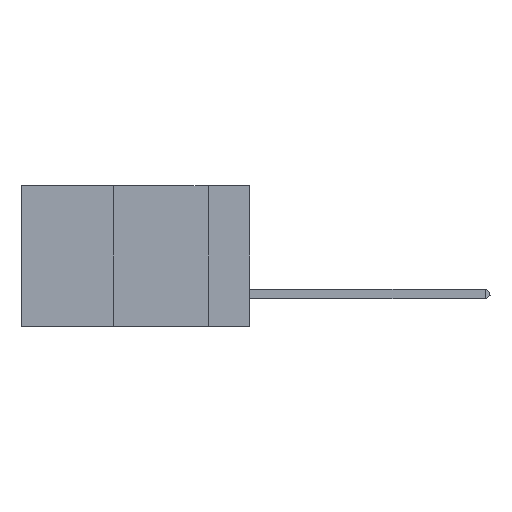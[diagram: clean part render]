
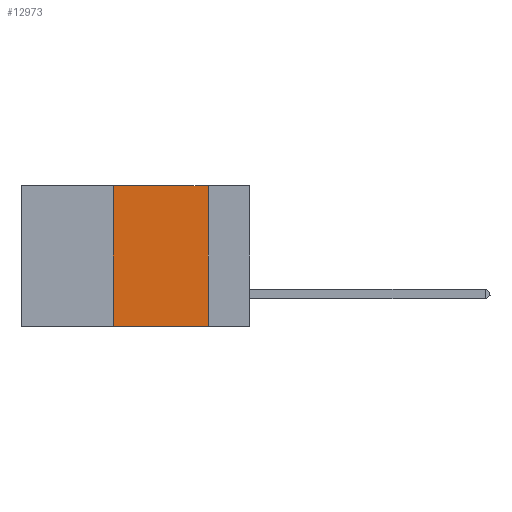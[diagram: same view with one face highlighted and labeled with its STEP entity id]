
A CAD part, left-side view. The second image highlights one B-rep face of the part: STEP entity #12973.
In plain terms, the highlighted planar face has unit normal (-1, 0, 0).
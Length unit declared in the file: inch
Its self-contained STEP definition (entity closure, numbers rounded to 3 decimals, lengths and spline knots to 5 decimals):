
#268 = ORIENTED_EDGE ( 'NONE', *, *, #5433, .F. ) ;
#937 = AXIS2_PLACEMENT_3D ( 'NONE', #36667, #13657, #36542 ) ;
#2885 = FACE_OUTER_BOUND ( 'NONE', #14887, .T. ) ;
#4518 = LINE ( 'NONE', #21459, #18249 ) ;
#5433 = EDGE_CURVE ( 'NONE', #33596, #33180, #33106, .T. ) ;
#8231 = DIRECTION ( 'NONE',  ( 0., 0., 1. ) ) ;
#8996 = CARTESIAN_POINT ( 'NONE',  ( 0., 0.6, -0.37 ) ) ;
#9204 = DIRECTION ( 'NONE',  ( 0., 0., -1. ) ) ;
#9628 = CARTESIAN_POINT ( 'NONE',  ( 0., 0.36, 0. ) ) ;
#11855 = VERTEX_POINT ( 'NONE', #20778 ) ;
#12973 = ADVANCED_FACE ( 'NONE', ( #2885 ), #30639, .F. ) ;
#13657 = DIRECTION ( 'NONE',  ( 1., 0., 0. ) ) ;
#14887 = EDGE_LOOP ( 'NONE', ( #19943, #26141, #268, #23049 ) ) ;
#16085 = VECTOR ( 'NONE', #9204, 39.37008 ) ;
#16979 = VERTEX_POINT ( 'NONE', #28825 ) ;
#18249 = VECTOR ( 'NONE', #24515, 39.37008 ) ;
#19943 = ORIENTED_EDGE ( 'NONE', *, *, #33631, .F. ) ;
#20144 = VECTOR ( 'NONE', #29435, 39.37008 ) ;
#20778 = CARTESIAN_POINT ( 'NONE',  ( 0., 0.11, -0.37 ) ) ;
#21459 = CARTESIAN_POINT ( 'NONE',  ( 0., 0.6, 0. ) ) ;
#23049 = ORIENTED_EDGE ( 'NONE', *, *, #28765, .T. ) ;
#23074 = CARTESIAN_POINT ( 'NONE',  ( 0., 0.36, -0.37 ) ) ;
#24368 = EDGE_CURVE ( 'NONE', #33180, #16979, #4518, .T. ) ;
#24515 = DIRECTION ( 'NONE',  ( 0., -1., 0. ) ) ;
#26141 = ORIENTED_EDGE ( 'NONE', *, *, #24368, .F. ) ;
#26164 = CARTESIAN_POINT ( 'NONE',  ( 0., 0.36, 0. ) ) ;
#26307 = VECTOR ( 'NONE', #8231, 39.37008 ) ;
#26871 = CARTESIAN_POINT ( 'NONE',  ( 0., 0.11, 0. ) ) ;
#28765 = EDGE_CURVE ( 'NONE', #33596, #11855, #29697, .T. ) ;
#28825 = CARTESIAN_POINT ( 'NONE',  ( 0., 0.11, 0. ) ) ;
#29435 = DIRECTION ( 'NONE',  ( 0., -1., 0. ) ) ;
#29697 = LINE ( 'NONE', #8996, #20144 ) ;
#30639 = PLANE ( 'NONE',  #937 ) ;
#33106 = LINE ( 'NONE', #26164, #26307 ) ;
#33180 = VERTEX_POINT ( 'NONE', #9628 ) ;
#33596 = VERTEX_POINT ( 'NONE', #23074 ) ;
#33631 = EDGE_CURVE ( 'NONE', #16979, #11855, #36659, .T. ) ;
#36542 = DIRECTION ( 'NONE',  ( 0., 0., -1. ) ) ;
#36659 = LINE ( 'NONE', #26871, #16085 ) ;
#36667 = CARTESIAN_POINT ( 'NONE',  ( 0., 0.6, 0. ) ) ;
